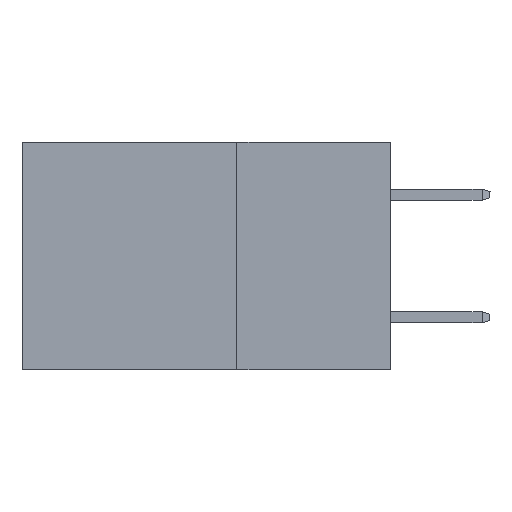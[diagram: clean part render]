
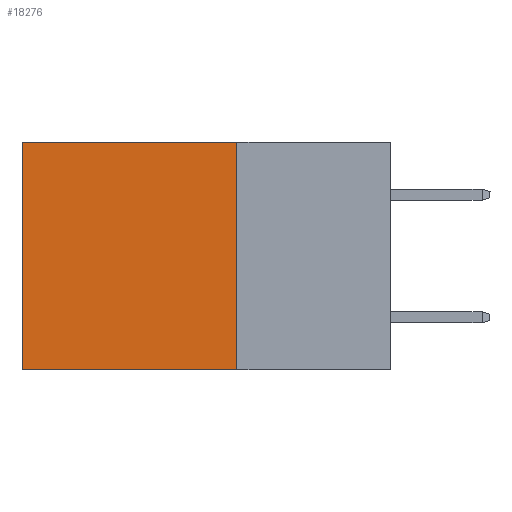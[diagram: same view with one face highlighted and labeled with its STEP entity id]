
A CAD part, left-side view. The second image highlights one B-rep face of the part: STEP entity #18276.
In plain terms, the highlighted planar face has unit normal (-1, 0, 0).
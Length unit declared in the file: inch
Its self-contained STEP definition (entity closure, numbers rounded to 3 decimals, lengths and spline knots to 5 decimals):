
#207 = LINE ( 'NONE', #6233, #16711 ) ;
#1113 = EDGE_LOOP ( 'NONE', ( #8166, #15054, #9023, #14276 ) ) ;
#2087 = EDGE_CURVE ( 'NONE', #19371, #13469, #207, .T. ) ;
#4063 = VECTOR ( 'NONE', #12618, 39.37008 ) ;
#4346 = VERTEX_POINT ( 'NONE', #13717 ) ;
#4564 = EDGE_CURVE ( 'NONE', #8721, #19371, #16583, .T. ) ;
#5707 = DIRECTION ( 'NONE',  ( 0., 0., -1. ) ) ;
#5779 = DIRECTION ( 'NONE',  ( 1., 0., 0. ) ) ;
#5843 = CARTESIAN_POINT ( 'NONE',  ( 0.2875, 0.25, -0.37 ) ) ;
#5932 = PLANE ( 'NONE',  #8328 ) ;
#6233 = CARTESIAN_POINT ( 'NONE',  ( 0.2875, 0.25, -0.37 ) ) ;
#7092 = EDGE_CURVE ( 'NONE', #8721, #4346, #11581, .T. ) ;
#7222 = CARTESIAN_POINT ( 'NONE',  ( 0.2875, 0.6, 0. ) ) ;
#8166 = ORIENTED_EDGE ( 'NONE', *, *, #20348, .T. ) ;
#8328 = AXIS2_PLACEMENT_3D ( 'NONE', #20153, #5779, #5707 ) ;
#8721 = VERTEX_POINT ( 'NONE', #18792 ) ;
#9023 = ORIENTED_EDGE ( 'NONE', *, *, #4564, .F. ) ;
#9061 = FACE_OUTER_BOUND ( 'NONE', #1113, .T. ) ;
#11281 = DIRECTION ( 'NONE',  ( 0., 1., 0. ) ) ;
#11581 = LINE ( 'NONE', #14217, #4063 ) ;
#12106 = DIRECTION ( 'NONE',  ( 0., 0., -1. ) ) ;
#12618 = DIRECTION ( 'NONE',  ( 0., 1., 0. ) ) ;
#13469 = VERTEX_POINT ( 'NONE', #19531 ) ;
#13717 = CARTESIAN_POINT ( 'NONE',  ( 0.2875, 0.6, 0. ) ) ;
#14217 = CARTESIAN_POINT ( 'NONE',  ( 0.2875, 0.25, 0. ) ) ;
#14262 = DIRECTION ( 'NONE',  ( 0., 0., -1. ) ) ;
#14276 = ORIENTED_EDGE ( 'NONE', *, *, #7092, .T. ) ;
#15034 = LINE ( 'NONE', #7222, #17287 ) ;
#15054 = ORIENTED_EDGE ( 'NONE', *, *, #2087, .F. ) ;
#16583 = LINE ( 'NONE', #19195, #17849 ) ;
#16711 = VECTOR ( 'NONE', #11281, 39.37008 ) ;
#17287 = VECTOR ( 'NONE', #12106, 39.37008 ) ;
#17849 = VECTOR ( 'NONE', #14262, 39.37008 ) ;
#18276 = ADVANCED_FACE ( 'NONE', ( #9061 ), #5932, .F. ) ;
#18792 = CARTESIAN_POINT ( 'NONE',  ( 0.2875, 0.25, 0. ) ) ;
#19195 = CARTESIAN_POINT ( 'NONE',  ( 0.2875, 0.25, 0. ) ) ;
#19371 = VERTEX_POINT ( 'NONE', #5843 ) ;
#19531 = CARTESIAN_POINT ( 'NONE',  ( 0.2875, 0.6, -0.37 ) ) ;
#20153 = CARTESIAN_POINT ( 'NONE',  ( 0.2875, 0.25, 0. ) ) ;
#20348 = EDGE_CURVE ( 'NONE', #4346, #13469, #15034, .T. ) ;
